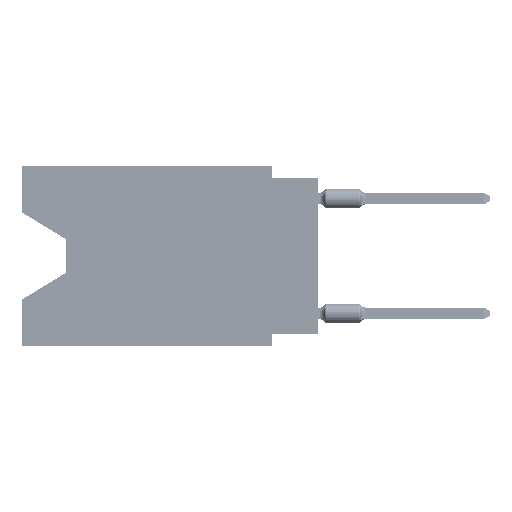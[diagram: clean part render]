
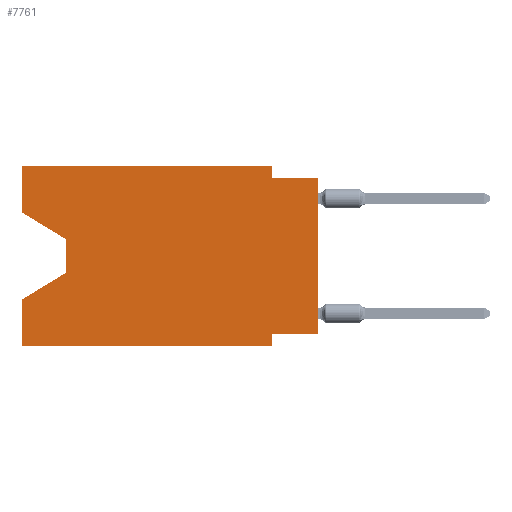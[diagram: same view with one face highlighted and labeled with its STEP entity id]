
A CAD part, left-side view. The second image highlights one B-rep face of the part: STEP entity #7761.
In plain terms, the highlighted planar face has unit normal (-1, 0, 0).
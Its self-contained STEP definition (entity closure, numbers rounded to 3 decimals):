
#146 = EDGE_CURVE ( 'NONE', #56396, #52323, #17685, .T. ) ;
#247 = ORIENTED_EDGE ( 'NONE', *, *, #146, .F. ) ;
#550 = ORIENTED_EDGE ( 'NONE', *, *, #50736, .F. ) ;
#1634 = ORIENTED_EDGE ( 'NONE', *, *, #59763, .F. ) ;
#1736 = CARTESIAN_POINT ( 'NONE',  ( 0., 13.97, -4.013 ) ) ;
#2754 = EDGE_CURVE ( 'NONE', #62061, #37059, #19466, .T. ) ;
#4224 = LINE ( 'NONE', #66710, #30657 ) ;
#4645 = ORIENTED_EDGE ( 'NONE', *, *, #23059, .F. ) ;
#5114 = CARTESIAN_POINT ( 'NONE',  ( 0., 13.97, -5.893 ) ) ;
#5474 = DIRECTION ( 'NONE',  ( 0., 0., 1. ) ) ;
#7761 = ADVANCED_FACE ( 'NONE', ( #59786 ), #10718, .F. ) ;
#9419 = CARTESIAN_POINT ( 'NONE',  ( 0., 16.383, 0. ) ) ;
#10550 = ORIENTED_EDGE ( 'NONE', *, *, #18741, .F. ) ;
#10718 = PLANE ( 'NONE',  #69335 ) ;
#11054 = CARTESIAN_POINT ( 'NONE',  ( 0., 16.383, 0. ) ) ;
#17685 = LINE ( 'NONE', #68216, #49010 ) ;
#18741 = EDGE_CURVE ( 'NONE', #44174, #56396, #71287, .T. ) ;
#18787 = DIRECTION ( 'NONE',  ( 0., 0., -1. ) ) ;
#18917 = DIRECTION ( 'NONE',  ( 0., -1., 0. ) ) ;
#19466 = LINE ( 'NONE', #41643, #65496 ) ;
#19545 = CARTESIAN_POINT ( 'NONE',  ( 0., 13.97, -5.893 ) ) ;
#21793 = ORIENTED_EDGE ( 'NONE', *, *, #56556, .T. ) ;
#22180 = LINE ( 'NONE', #33797, #65504 ) ;
#22543 = CARTESIAN_POINT ( 'NONE',  ( 0., 16.383, 0. ) ) ;
#23059 = EDGE_CURVE ( 'NONE', #27337, #35596, #61552, .T. ) ;
#23526 = ORIENTED_EDGE ( 'NONE', *, *, #65886, .F. ) ;
#23906 = ORIENTED_EDGE ( 'NONE', *, *, #35192, .T. ) ;
#24908 = DIRECTION ( 'NONE',  ( 0., 0., -1. ) ) ;
#26542 = VERTEX_POINT ( 'NONE', #63148 ) ;
#26848 = CARTESIAN_POINT ( 'NONE',  ( 0., 16.383, -7.36 ) ) ;
#27337 = VERTEX_POINT ( 'NONE', #70124 ) ;
#30657 = VECTOR ( 'NONE', #60169, 1000. ) ;
#31096 = VERTEX_POINT ( 'NONE', #41873 ) ;
#31184 = VERTEX_POINT ( 'NONE', #68777 ) ;
#32894 = DIRECTION ( 'NONE',  ( 1., 0., 0. ) ) ;
#33109 = LINE ( 'NONE', #55270, #44728 ) ;
#33797 = CARTESIAN_POINT ( 'NONE',  ( 0., 2.54, 0. ) ) ;
#34019 = CARTESIAN_POINT ( 'NONE',  ( 0., 2.54, -9.271 ) ) ;
#35192 = EDGE_CURVE ( 'NONE', #37123, #35596, #71617, .T. ) ;
#35596 = VERTEX_POINT ( 'NONE', #26848 ) ;
#37059 = VERTEX_POINT ( 'NONE', #1736 ) ;
#37123 = VERTEX_POINT ( 'NONE', #19545 ) ;
#38057 = EDGE_LOOP ( 'NONE', ( #56914, #21793, #23906, #4645, #54176, #247, #10550, #68563, #23526, #1634, #46583, #550 ) ) ;
#38640 = EDGE_CURVE ( 'NONE', #27337, #52323, #4224, .T. ) ;
#39439 = VECTOR ( 'NONE', #70616, 1000. ) ;
#39472 = VECTOR ( 'NONE', #51239, 1000. ) ;
#39626 = DIRECTION ( 'NONE',  ( 0., 0.855, -0.519 ) ) ;
#40113 = VECTOR ( 'NONE', #18917, 1000. ) ;
#41305 = CARTESIAN_POINT ( 'NONE',  ( 0., 0., -0.635 ) ) ;
#41643 = CARTESIAN_POINT ( 'NONE',  ( 0., 16.383, -2.546 ) ) ;
#41873 = CARTESIAN_POINT ( 'NONE',  ( 0., 0., -0.635 ) ) ;
#42091 = VECTOR ( 'NONE', #60476, 1000. ) ;
#43158 = CARTESIAN_POINT ( 'NONE',  ( 0., 16.383, -2.546 ) ) ;
#44174 = VERTEX_POINT ( 'NONE', #50173 ) ;
#44364 = VERTEX_POINT ( 'NONE', #9419 ) ;
#44380 = CARTESIAN_POINT ( 'NONE',  ( 0., 0., -9.271 ) ) ;
#44728 = VECTOR ( 'NONE', #5474, 1000. ) ;
#46150 = VECTOR ( 'NONE', #24908, 1000. ) ;
#46583 = ORIENTED_EDGE ( 'NONE', *, *, #54620, .F. ) ;
#47329 = CARTESIAN_POINT ( 'NONE',  ( 0., 2.54, -9.906 ) ) ;
#47434 = CARTESIAN_POINT ( 'NONE',  ( 0., 13.97, -4.013 ) ) ;
#48178 = CARTESIAN_POINT ( 'NONE',  ( 0., 16.383, 0. ) ) ;
#49010 = VECTOR ( 'NONE', #18787, 1000. ) ;
#50173 = CARTESIAN_POINT ( 'NONE',  ( 0., 0., -9.271 ) ) ;
#50196 = DIRECTION ( 'NONE',  ( 0., 1., 0. ) ) ;
#50736 = EDGE_CURVE ( 'NONE', #62061, #44364, #67962, .T. ) ;
#51239 = DIRECTION ( 'NONE',  ( 0., 0., 1. ) ) ;
#52323 = VERTEX_POINT ( 'NONE', #47329 ) ;
#54176 = ORIENTED_EDGE ( 'NONE', *, *, #38640, .T. ) ;
#54368 = EDGE_CURVE ( 'NONE', #44174, #31096, #33109, .T. ) ;
#54620 = EDGE_CURVE ( 'NONE', #44364, #31184, #64681, .T. ) ;
#55270 = CARTESIAN_POINT ( 'NONE',  ( 0., 0., 0. ) ) ;
#55793 = VECTOR ( 'NONE', #50196, 1000. ) ;
#55851 = VECTOR ( 'NONE', #39626, 1000. ) ;
#56396 = VERTEX_POINT ( 'NONE', #34019 ) ;
#56556 = EDGE_CURVE ( 'NONE', #37059, #37123, #63083, .T. ) ;
#56914 = ORIENTED_EDGE ( 'NONE', *, *, #2754, .T. ) ;
#59763 = EDGE_CURVE ( 'NONE', #31184, #26542, #22180, .T. ) ;
#59786 = FACE_OUTER_BOUND ( 'NONE', #38057, .T. ) ;
#60169 = DIRECTION ( 'NONE',  ( 0., -1., 0. ) ) ;
#60476 = DIRECTION ( 'NONE',  ( 0., 0., 1. ) ) ;
#61552 = LINE ( 'NONE', #11054, #42091 ) ;
#62061 = VERTEX_POINT ( 'NONE', #43158 ) ;
#63083 = LINE ( 'NONE', #47434, #46150 ) ;
#63148 = CARTESIAN_POINT ( 'NONE',  ( 0., 2.54, -0.635 ) ) ;
#63799 = DIRECTION ( 'NONE',  ( 0., -0.855, -0.519 ) ) ;
#64681 = LINE ( 'NONE', #68705, #40113 ) ;
#65168 = LINE ( 'NONE', #41305, #39439 ) ;
#65256 = DIRECTION ( 'NONE',  ( 0., 0., -1. ) ) ;
#65496 = VECTOR ( 'NONE', #63799, 1000. ) ;
#65504 = VECTOR ( 'NONE', #66518, 1000. ) ;
#65886 = EDGE_CURVE ( 'NONE', #26542, #31096, #65168, .T. ) ;
#66518 = DIRECTION ( 'NONE',  ( 0., 0., -1. ) ) ;
#66710 = CARTESIAN_POINT ( 'NONE',  ( 0., 16.383, -9.906 ) ) ;
#67962 = LINE ( 'NONE', #22543, #39472 ) ;
#68216 = CARTESIAN_POINT ( 'NONE',  ( 0., 2.54, -9.906 ) ) ;
#68563 = ORIENTED_EDGE ( 'NONE', *, *, #54368, .T. ) ;
#68705 = CARTESIAN_POINT ( 'NONE',  ( 0., 16.383, 0. ) ) ;
#68777 = CARTESIAN_POINT ( 'NONE',  ( 0., 2.54, 0. ) ) ;
#69335 = AXIS2_PLACEMENT_3D ( 'NONE', #48178, #32894, #65256 ) ;
#70124 = CARTESIAN_POINT ( 'NONE',  ( 0., 16.383, -9.906 ) ) ;
#70616 = DIRECTION ( 'NONE',  ( 0., -1., 0. ) ) ;
#71287 = LINE ( 'NONE', #44380, #55793 ) ;
#71617 = LINE ( 'NONE', #5114, #55851 ) ;
